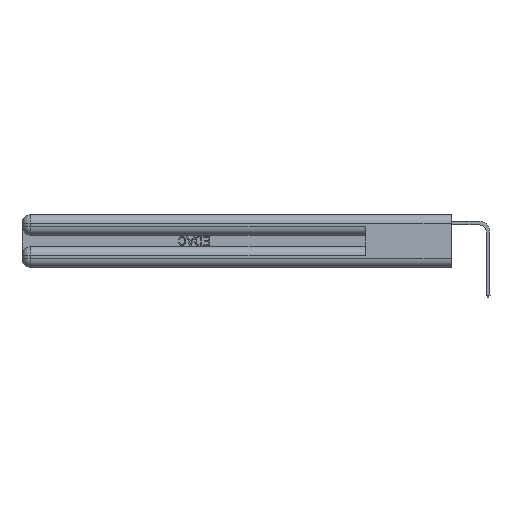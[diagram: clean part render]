
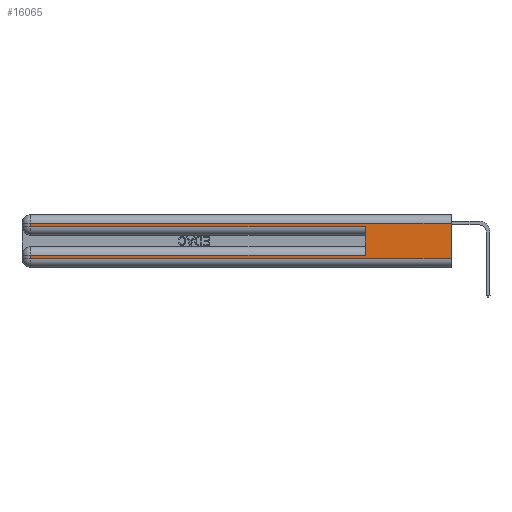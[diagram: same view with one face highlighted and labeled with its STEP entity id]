
A CAD part, left-side view. The second image highlights one B-rep face of the part: STEP entity #16065.
In plain terms, the highlighted planar face has unit normal (-1, 0, 0).
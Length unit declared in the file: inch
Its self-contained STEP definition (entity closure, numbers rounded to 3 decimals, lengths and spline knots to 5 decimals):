
#461 = LINE ( 'NONE', #13389, #18044 ) ;
#1035 = EDGE_CURVE ( 'NONE', #19026, #9717, #2683, .T. ) ;
#1717 = AXIS2_PLACEMENT_3D ( 'NONE', #27324, #18969, #16979 ) ;
#1860 = ORIENTED_EDGE ( 'NONE', *, *, #6297, .T. ) ;
#2683 = LINE ( 'NONE', #26689, #5271 ) ;
#2705 = DIRECTION ( 'NONE',  ( 0., 0., 1. ) ) ;
#2879 = DIRECTION ( 'NONE',  ( 0., 1., 0. ) ) ;
#3047 = VERTEX_POINT ( 'NONE', #23784 ) ;
#3269 = VERTEX_POINT ( 'NONE', #20385 ) ;
#4161 = VERTEX_POINT ( 'NONE', #23729 ) ;
#4730 = EDGE_CURVE ( 'NONE', #3269, #26803, #26773, .T. ) ;
#5227 = ORIENTED_EDGE ( 'NONE', *, *, #24576, .T. ) ;
#5271 = VECTOR ( 'NONE', #7321, 39.37008 ) ;
#5395 = VERTEX_POINT ( 'NONE', #14269 ) ;
#6297 = EDGE_CURVE ( 'NONE', #19026, #4161, #21687, .T. ) ;
#6470 = VECTOR ( 'NONE', #16813, 39.37008 ) ;
#7321 = DIRECTION ( 'NONE',  ( 0., 0., -1. ) ) ;
#9015 = ORIENTED_EDGE ( 'NONE', *, *, #18806, .T. ) ;
#9717 = VERTEX_POINT ( 'NONE', #16996 ) ;
#10011 = ORIENTED_EDGE ( 'NONE', *, *, #23911, .T. ) ;
#11061 = DIRECTION ( 'NONE',  ( 0., 0., -1. ) ) ;
#11525 = CARTESIAN_POINT ( 'NONE',  ( 0., 2.94, 0.37 ) ) ;
#11921 = ORIENTED_EDGE ( 'NONE', *, *, #23449, .T. ) ;
#11935 = DIRECTION ( 'NONE',  ( 0., 0., -1. ) ) ;
#12346 = PLANE ( 'NONE',  #1717 ) ;
#12975 = EDGE_LOOP ( 'NONE', ( #17616, #1860, #9015, #11921, #20143, #20837, #5227, #10011 ) ) ;
#13389 = CARTESIAN_POINT ( 'NONE',  ( 0., 0.6, 0.145 ) ) ;
#13724 = CARTESIAN_POINT ( 'NONE',  ( 0., 2.94, 0.37 ) ) ;
#13869 = CARTESIAN_POINT ( 'NONE',  ( 0., 0., 0.31 ) ) ;
#14039 = CARTESIAN_POINT ( 'NONE',  ( 0., 0., 0.285 ) ) ;
#14269 = CARTESIAN_POINT ( 'NONE',  ( 0., 2.94, 0.06 ) ) ;
#14305 = DIRECTION ( 'NONE',  ( 0., 1., 0. ) ) ;
#14313 = LINE ( 'NONE', #14039, #19073 ) ;
#14371 = VECTOR ( 'NONE', #11061, 39.37008 ) ;
#14523 = VECTOR ( 'NONE', #11935, 39.37008 ) ;
#16065 = ADVANCED_FACE ( 'NONE', ( #21380 ), #12346, .F. ) ;
#16813 = DIRECTION ( 'NONE',  ( 0., -1., 0. ) ) ;
#16979 = DIRECTION ( 'NONE',  ( 0., 0., -1. ) ) ;
#16996 = CARTESIAN_POINT ( 'NONE',  ( 0., 0., 0.06 ) ) ;
#17252 = VECTOR ( 'NONE', #2879, 39.37008 ) ;
#17616 = ORIENTED_EDGE ( 'NONE', *, *, #1035, .F. ) ;
#18044 = VECTOR ( 'NONE', #2705, 39.37008 ) ;
#18806 = EDGE_CURVE ( 'NONE', #4161, #3047, #24188, .T. ) ;
#18969 = DIRECTION ( 'NONE',  ( 1., 0., 0. ) ) ;
#18975 = VECTOR ( 'NONE', #14305, 39.37008 ) ;
#19026 = VERTEX_POINT ( 'NONE', #13869 ) ;
#19073 = VECTOR ( 'NONE', #22662, 39.37008 ) ;
#19490 = CARTESIAN_POINT ( 'NONE',  ( 0., 0., 0.06 ) ) ;
#19983 = LINE ( 'NONE', #11525, #14523 ) ;
#20143 = ORIENTED_EDGE ( 'NONE', *, *, #20649, .F. ) ;
#20385 = CARTESIAN_POINT ( 'NONE',  ( 0., 0.6, 0.085 ) ) ;
#20649 = EDGE_CURVE ( 'NONE', #3269, #23342, #461, .T. ) ;
#20837 = ORIENTED_EDGE ( 'NONE', *, *, #4730, .T. ) ;
#21380 = FACE_OUTER_BOUND ( 'NONE', #12975, .T. ) ;
#21687 = LINE ( 'NONE', #25925, #17252 ) ;
#22239 = CARTESIAN_POINT ( 'NONE',  ( 0., 0.6, 0.285 ) ) ;
#22662 = DIRECTION ( 'NONE',  ( 0., -1., 0. ) ) ;
#23329 = LINE ( 'NONE', #19490, #6470 ) ;
#23342 = VERTEX_POINT ( 'NONE', #22239 ) ;
#23449 = EDGE_CURVE ( 'NONE', #3047, #23342, #14313, .T. ) ;
#23450 = CARTESIAN_POINT ( 'NONE',  ( 0., 2.94, 0.085 ) ) ;
#23729 = CARTESIAN_POINT ( 'NONE',  ( 0., 2.94, 0.31 ) ) ;
#23784 = CARTESIAN_POINT ( 'NONE',  ( 0., 2.94, 0.285 ) ) ;
#23911 = EDGE_CURVE ( 'NONE', #5395, #9717, #23329, .T. ) ;
#24188 = LINE ( 'NONE', #13724, #14371 ) ;
#24576 = EDGE_CURVE ( 'NONE', #26803, #5395, #19983, .T. ) ;
#25925 = CARTESIAN_POINT ( 'NONE',  ( 0., 0., 0.31 ) ) ;
#26689 = CARTESIAN_POINT ( 'NONE',  ( 0., 0., 0.37 ) ) ;
#26773 = LINE ( 'NONE', #27053, #18975 ) ;
#26803 = VERTEX_POINT ( 'NONE', #23450 ) ;
#27053 = CARTESIAN_POINT ( 'NONE',  ( 0., 0., 0.085 ) ) ;
#27324 = CARTESIAN_POINT ( 'NONE',  ( 0., 0., 0.37 ) ) ;
